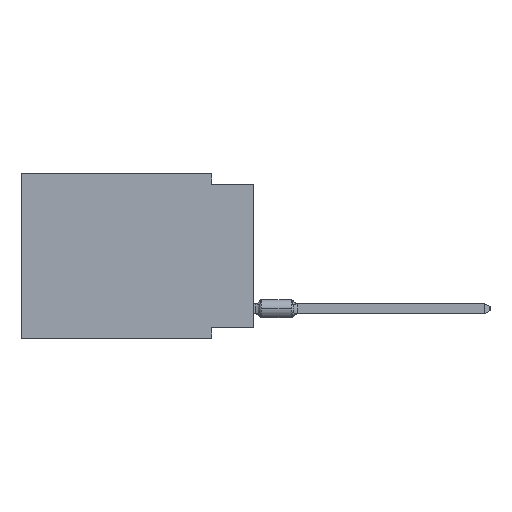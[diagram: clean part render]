
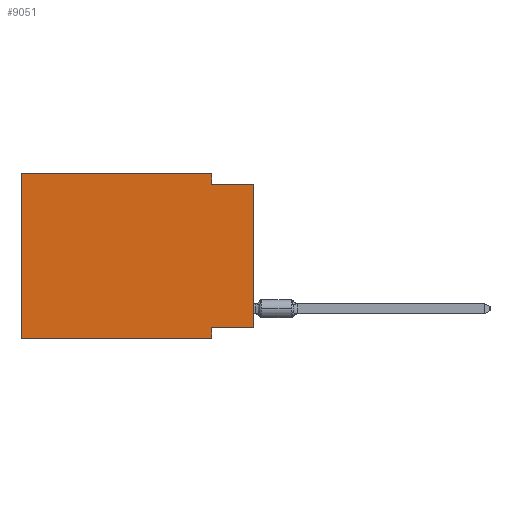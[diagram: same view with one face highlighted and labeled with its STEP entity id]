
A CAD part, left-side view. The second image highlights one B-rep face of the part: STEP entity #9051.
In plain terms, the highlighted planar face has unit normal (-1, 0, 0).
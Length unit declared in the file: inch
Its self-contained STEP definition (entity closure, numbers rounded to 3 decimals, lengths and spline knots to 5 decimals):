
#202 = VERTEX_POINT ( 'NONE', #23559 ) ;
#664 = VECTOR ( 'NONE', #56831, 39.37008 ) ;
#940 = CARTESIAN_POINT ( 'NONE',  ( 0., 0.1, -0.39 ) ) ;
#1893 = CARTESIAN_POINT ( 'NONE',  ( 0., 0., -0.365 ) ) ;
#2043 = ORIENTED_EDGE ( 'NONE', *, *, #12605, .F. ) ;
#3067 = DIRECTION ( 'NONE',  ( 0., 0., -1. ) ) ;
#3287 = VECTOR ( 'NONE', #50228, 39.37008 ) ;
#3970 = DIRECTION ( 'NONE',  ( 0., 0., 1. ) ) ;
#4718 = CARTESIAN_POINT ( 'NONE',  ( 0., 0.55, -0.39 ) ) ;
#5401 = DIRECTION ( 'NONE',  ( 0., 0., 1. ) ) ;
#6434 = VERTEX_POINT ( 'NONE', #14610 ) ;
#6645 = ORIENTED_EDGE ( 'NONE', *, *, #28586, .F. ) ;
#7500 = VERTEX_POINT ( 'NONE', #39577 ) ;
#7744 = PLANE ( 'NONE',  #34339 ) ;
#8445 = CARTESIAN_POINT ( 'NONE',  ( 0., 0., -0.025 ) ) ;
#9051 = ADVANCED_FACE ( 'NONE', ( #38819 ), #7744, .F. ) ;
#9121 = DIRECTION ( 'NONE',  ( 0., -1., 0. ) ) ;
#12605 = EDGE_CURVE ( 'NONE', #202, #51560, #15360, .T. ) ;
#13517 = LINE ( 'NONE', #4718, #26490 ) ;
#14610 = CARTESIAN_POINT ( 'NONE',  ( 0., 0.55, 0. ) ) ;
#15360 = LINE ( 'NONE', #1893, #41299 ) ;
#17119 = DIRECTION ( 'NONE',  ( 1., 0., 0. ) ) ;
#18399 = VECTOR ( 'NONE', #22410, 39.37008 ) ;
#18806 = DIRECTION ( 'NONE',  ( 0., 0., -1. ) ) ;
#18844 = LINE ( 'NONE', #36134, #3287 ) ;
#19064 = EDGE_CURVE ( 'NONE', #52383, #40087, #13517, .T. ) ;
#20489 = VECTOR ( 'NONE', #18806, 39.37008 ) ;
#21506 = CARTESIAN_POINT ( 'NONE',  ( 0., 0.55, 0. ) ) ;
#22410 = DIRECTION ( 'NONE',  ( 0., 0., -1. ) ) ;
#23253 = CARTESIAN_POINT ( 'NONE',  ( 0., 0.1, -0.39 ) ) ;
#23559 = CARTESIAN_POINT ( 'NONE',  ( 0., 0., -0.365 ) ) ;
#24241 = ORIENTED_EDGE ( 'NONE', *, *, #25849, .F. ) ;
#24538 = CARTESIAN_POINT ( 'NONE',  ( 0., 0.55, -0.39 ) ) ;
#24542 = VERTEX_POINT ( 'NONE', #24545 ) ;
#24545 = CARTESIAN_POINT ( 'NONE',  ( 0., 0., -0.025 ) ) ;
#25849 = EDGE_CURVE ( 'NONE', #7500, #24542, #30691, .T. ) ;
#26299 = ORIENTED_EDGE ( 'NONE', *, *, #28361, .F. ) ;
#26490 = VECTOR ( 'NONE', #9121, 39.37008 ) ;
#27084 = LINE ( 'NONE', #45549, #28194 ) ;
#28194 = VECTOR ( 'NONE', #5401, 39.37008 ) ;
#28361 = EDGE_CURVE ( 'NONE', #52383, #6434, #35311, .T. ) ;
#28586 = EDGE_CURVE ( 'NONE', #48750, #7500, #41151, .T. ) ;
#30691 = LINE ( 'NONE', #8445, #664 ) ;
#31872 = ORIENTED_EDGE ( 'NONE', *, *, #33009, .F. ) ;
#33009 = EDGE_CURVE ( 'NONE', #51560, #40087, #41089, .T. ) ;
#34339 = AXIS2_PLACEMENT_3D ( 'NONE', #21506, #17119, #3067 ) ;
#34412 = EDGE_CURVE ( 'NONE', #202, #24542, #27084, .T. ) ;
#35311 = LINE ( 'NONE', #47650, #45518 ) ;
#35599 = ORIENTED_EDGE ( 'NONE', *, *, #34412, .T. ) ;
#36134 = CARTESIAN_POINT ( 'NONE',  ( 0., 0.55, 0. ) ) ;
#38228 = CARTESIAN_POINT ( 'NONE',  ( 0., 0.1, -0.365 ) ) ;
#38506 = DIRECTION ( 'NONE',  ( 0., 1., 0. ) ) ;
#38819 = FACE_OUTER_BOUND ( 'NONE', #48146, .T. ) ;
#38953 = EDGE_CURVE ( 'NONE', #6434, #48750, #18844, .T. ) ;
#39577 = CARTESIAN_POINT ( 'NONE',  ( 0., 0.1, -0.025 ) ) ;
#40087 = VERTEX_POINT ( 'NONE', #23253 ) ;
#41089 = LINE ( 'NONE', #940, #20489 ) ;
#41151 = LINE ( 'NONE', #49951, #18399 ) ;
#41299 = VECTOR ( 'NONE', #38506, 39.37008 ) ;
#42890 = ORIENTED_EDGE ( 'NONE', *, *, #19064, .T. ) ;
#45518 = VECTOR ( 'NONE', #3970, 39.37008 ) ;
#45549 = CARTESIAN_POINT ( 'NONE',  ( 0., 0., 0. ) ) ;
#47650 = CARTESIAN_POINT ( 'NONE',  ( 0., 0.55, 0. ) ) ;
#48146 = EDGE_LOOP ( 'NONE', ( #35599, #24241, #6645, #49014, #26299, #42890, #31872, #2043 ) ) ;
#48750 = VERTEX_POINT ( 'NONE', #51663 ) ;
#49014 = ORIENTED_EDGE ( 'NONE', *, *, #38953, .F. ) ;
#49951 = CARTESIAN_POINT ( 'NONE',  ( 0., 0.1, 0. ) ) ;
#50228 = DIRECTION ( 'NONE',  ( 0., -1., 0. ) ) ;
#51560 = VERTEX_POINT ( 'NONE', #38228 ) ;
#51663 = CARTESIAN_POINT ( 'NONE',  ( 0., 0.1, 0. ) ) ;
#52383 = VERTEX_POINT ( 'NONE', #24538 ) ;
#56831 = DIRECTION ( 'NONE',  ( 0., -1., 0. ) ) ;
